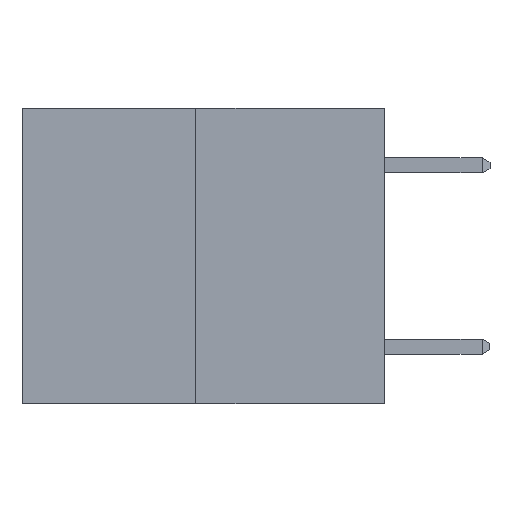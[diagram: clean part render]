
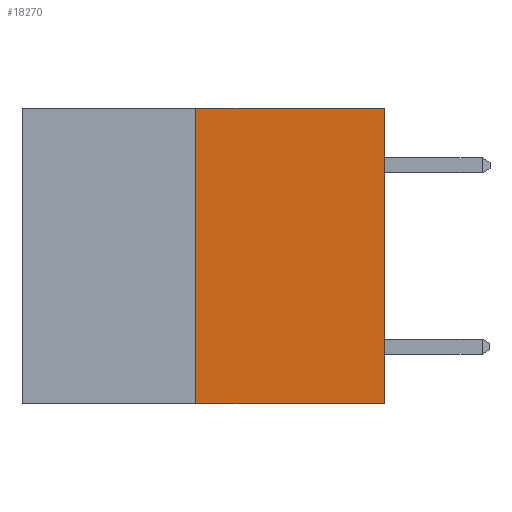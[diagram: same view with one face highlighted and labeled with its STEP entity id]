
A CAD part, left-side view. The second image highlights one B-rep face of the part: STEP entity #18270.
In plain terms, the highlighted planar face has unit normal (-1, 0, 0).
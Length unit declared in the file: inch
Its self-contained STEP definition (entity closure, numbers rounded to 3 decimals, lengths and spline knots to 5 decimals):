
#1379 = FACE_OUTER_BOUND ( 'NONE', #17329, .T. ) ;
#1792 = DIRECTION ( 'NONE',  ( 0., -1., 0. ) ) ;
#2229 = VECTOR ( 'NONE', #1792, 39.37008 ) ;
#2373 = DIRECTION ( 'NONE',  ( 0., 0., 1. ) ) ;
#4240 = CARTESIAN_POINT ( 'NONE',  ( 0., 0., -0.49 ) ) ;
#4834 = CARTESIAN_POINT ( 'NONE',  ( 0., 0.6, -0.49 ) ) ;
#5945 = VERTEX_POINT ( 'NONE', #8941 ) ;
#6650 = VERTEX_POINT ( 'NONE', #12000 ) ;
#6887 = AXIS2_PLACEMENT_3D ( 'NONE', #9788, #13166, #17498 ) ;
#7529 = EDGE_CURVE ( 'NONE', #5945, #17095, #12172, .T. ) ;
#8296 = VECTOR ( 'NONE', #10797, 39.37008 ) ;
#8941 = CARTESIAN_POINT ( 'NONE',  ( 0., 0.312, -0.49 ) ) ;
#9788 = CARTESIAN_POINT ( 'NONE',  ( 0., 0.6, 0. ) ) ;
#10643 = CARTESIAN_POINT ( 'NONE',  ( 0., 0.6, 0. ) ) ;
#10658 = EDGE_CURVE ( 'NONE', #6650, #18152, #14139, .T. ) ;
#10797 = DIRECTION ( 'NONE',  ( 0., -1., 0. ) ) ;
#11173 = DIRECTION ( 'NONE',  ( 0., 0., 1. ) ) ;
#11476 = LINE ( 'NONE', #14276, #17458 ) ;
#12000 = CARTESIAN_POINT ( 'NONE',  ( 0., 0.312, 0. ) ) ;
#12172 = LINE ( 'NONE', #4834, #8296 ) ;
#12460 = CARTESIAN_POINT ( 'NONE',  ( 0., 0., 0. ) ) ;
#13166 = DIRECTION ( 'NONE',  ( 1., 0., 0. ) ) ;
#13640 = EDGE_CURVE ( 'NONE', #17095, #18152, #13934, .T. ) ;
#13934 = LINE ( 'NONE', #14141, #18962 ) ;
#14139 = LINE ( 'NONE', #10643, #2229 ) ;
#14141 = CARTESIAN_POINT ( 'NONE',  ( 0., 0., 0. ) ) ;
#14276 = CARTESIAN_POINT ( 'NONE',  ( 0., 0.312, -0.49 ) ) ;
#14483 = ORIENTED_EDGE ( 'NONE', *, *, #7529, .T. ) ;
#14989 = ORIENTED_EDGE ( 'NONE', *, *, #13640, .T. ) ;
#15496 = ORIENTED_EDGE ( 'NONE', *, *, #10658, .F. ) ;
#15685 = ORIENTED_EDGE ( 'NONE', *, *, #17668, .F. ) ;
#17095 = VERTEX_POINT ( 'NONE', #4240 ) ;
#17329 = EDGE_LOOP ( 'NONE', ( #15685, #14483, #14989, #15496 ) ) ;
#17458 = VECTOR ( 'NONE', #11173, 39.37008 ) ;
#17498 = DIRECTION ( 'NONE',  ( 0., 0., -1. ) ) ;
#17668 = EDGE_CURVE ( 'NONE', #5945, #6650, #11476, .T. ) ;
#18152 = VERTEX_POINT ( 'NONE', #12460 ) ;
#18270 = ADVANCED_FACE ( 'NONE', ( #1379 ), #18560, .F. ) ;
#18560 = PLANE ( 'NONE',  #6887 ) ;
#18962 = VECTOR ( 'NONE', #2373, 39.37008 ) ;
